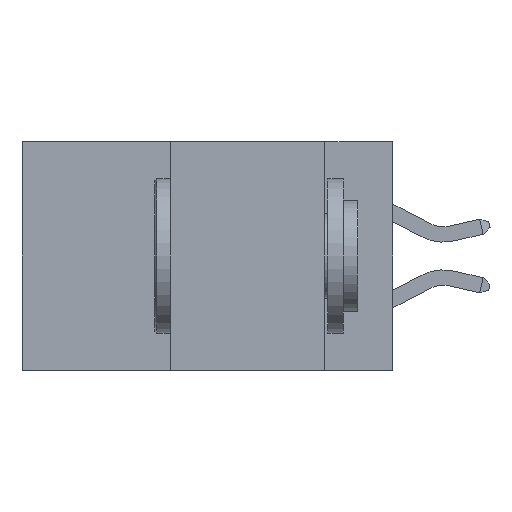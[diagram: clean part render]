
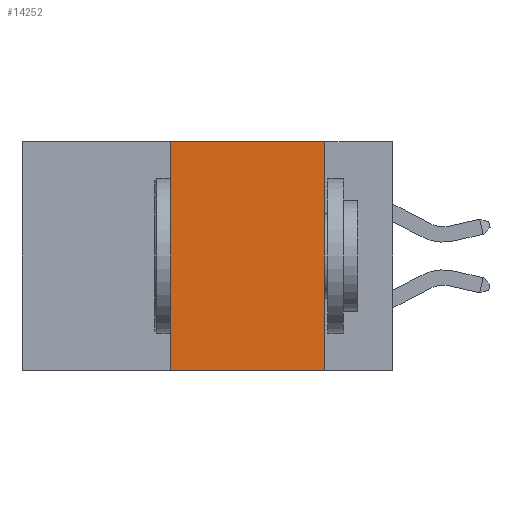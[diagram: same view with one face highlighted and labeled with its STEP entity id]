
A CAD part, left-side view. The second image highlights one B-rep face of the part: STEP entity #14252.
In plain terms, the highlighted planar face has unit normal (-1, 0, 0).
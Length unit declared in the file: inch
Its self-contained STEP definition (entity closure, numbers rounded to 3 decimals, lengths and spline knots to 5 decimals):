
#2099 = EDGE_LOOP ( 'NONE', ( #8316, #19987, #14805, #20107 ) ) ;
#2409 = FACE_OUTER_BOUND ( 'NONE', #2099, .T. ) ;
#3858 = VERTEX_POINT ( 'NONE', #7060 ) ;
#5114 = VERTEX_POINT ( 'NONE', #26236 ) ;
#5927 = DIRECTION ( 'NONE',  ( 0., -1., 0. ) ) ;
#6241 = CARTESIAN_POINT ( 'NONE',  ( 0., 0.6, 0. ) ) ;
#7060 = CARTESIAN_POINT ( 'NONE',  ( 0., 0.36, 0. ) ) ;
#7813 = LINE ( 'NONE', #15246, #22392 ) ;
#8316 = ORIENTED_EDGE ( 'NONE', *, *, #24723, .F. ) ;
#9640 = VECTOR ( 'NONE', #23278, 39.37008 ) ;
#11297 = CARTESIAN_POINT ( 'NONE',  ( 0., 0.6, 0. ) ) ;
#12957 = DIRECTION ( 'NONE',  ( 0., 0., 1. ) ) ;
#13425 = LINE ( 'NONE', #26731, #22999 ) ;
#13432 = DIRECTION ( 'NONE',  ( 1., 0., 0. ) ) ;
#14252 = ADVANCED_FACE ( 'NONE', ( #2409 ), #24226, .F. ) ;
#14805 = ORIENTED_EDGE ( 'NONE', *, *, #20687, .F. ) ;
#15246 = CARTESIAN_POINT ( 'NONE',  ( 0., 0.36, 0. ) ) ;
#15507 = AXIS2_PLACEMENT_3D ( 'NONE', #11297, #13432, #15721 ) ;
#15721 = DIRECTION ( 'NONE',  ( 0., 0., -1. ) ) ;
#16171 = EDGE_CURVE ( 'NONE', #3858, #23041, #22226, .T. ) ;
#17348 = CARTESIAN_POINT ( 'NONE',  ( 0., 0.11, 0. ) ) ;
#18781 = CARTESIAN_POINT ( 'NONE',  ( 0., 0.6, -0.37 ) ) ;
#19907 = EDGE_CURVE ( 'NONE', #5114, #20050, #22106, .T. ) ;
#19987 = ORIENTED_EDGE ( 'NONE', *, *, #16171, .F. ) ;
#20050 = VERTEX_POINT ( 'NONE', #21113 ) ;
#20107 = ORIENTED_EDGE ( 'NONE', *, *, #19907, .T. ) ;
#20687 = EDGE_CURVE ( 'NONE', #5114, #3858, #7813, .T. ) ;
#21113 = CARTESIAN_POINT ( 'NONE',  ( 0., 0.11, -0.37 ) ) ;
#22106 = LINE ( 'NONE', #18781, #27028 ) ;
#22226 = LINE ( 'NONE', #6241, #9640 ) ;
#22392 = VECTOR ( 'NONE', #12957, 39.37008 ) ;
#22999 = VECTOR ( 'NONE', #23072, 39.37008 ) ;
#23041 = VERTEX_POINT ( 'NONE', #17348 ) ;
#23072 = DIRECTION ( 'NONE',  ( 0., 0., -1. ) ) ;
#23278 = DIRECTION ( 'NONE',  ( 0., -1., 0. ) ) ;
#24226 = PLANE ( 'NONE',  #15507 ) ;
#24723 = EDGE_CURVE ( 'NONE', #23041, #20050, #13425, .T. ) ;
#26236 = CARTESIAN_POINT ( 'NONE',  ( 0., 0.36, -0.37 ) ) ;
#26731 = CARTESIAN_POINT ( 'NONE',  ( 0., 0.11, 0. ) ) ;
#27028 = VECTOR ( 'NONE', #5927, 39.37008 ) ;
